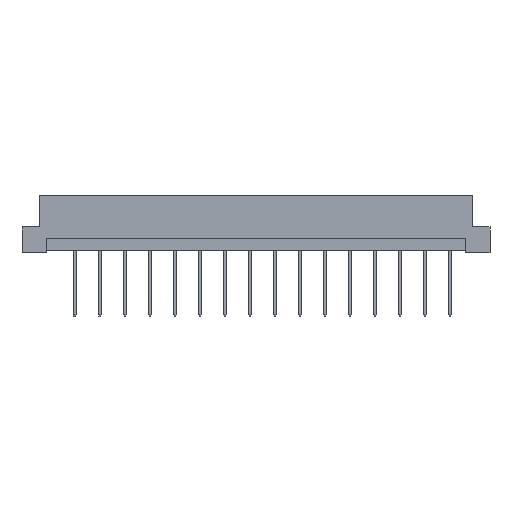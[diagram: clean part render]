
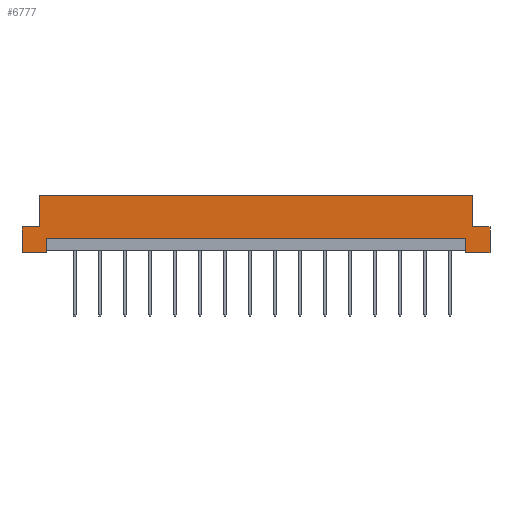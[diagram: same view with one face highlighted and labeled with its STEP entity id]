
A CAD part, front view. The second image highlights one B-rep face of the part: STEP entity #6777.
In plain terms, the highlighted planar face has unit normal (0, -1, 0).
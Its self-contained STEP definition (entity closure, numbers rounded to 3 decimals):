
#1 = VERTEX_POINT ( 'NONE', #7592 ) ;
#35 = EDGE_CURVE ( 'NONE', #4736, #4532, #8822, .T. ) ;
#127 = VERTEX_POINT ( 'NONE', #9904 ) ;
#182 = ORIENTED_EDGE ( 'NONE', *, *, #8289, .F. ) ;
#569 = LINE ( 'NONE', #14402, #5395 ) ;
#640 = VECTOR ( 'NONE', #4607, 1000. ) ;
#718 = VERTEX_POINT ( 'NONE', #14278 ) ;
#789 = DIRECTION ( 'NONE',  ( 0., 0., 1. ) ) ;
#864 = CARTESIAN_POINT ( 'NONE',  ( 44., 0., 5.2 ) ) ;
#945 = EDGE_CURVE ( 'NONE', #718, #7677, #9949, .T. ) ;
#1188 = CARTESIAN_POINT ( 'NONE',  ( -44., 0., 5.2 ) ) ;
#1294 = CARTESIAN_POINT ( 'NONE',  ( -47.5, 0., 0. ) ) ;
#1358 = CARTESIAN_POINT ( 'NONE',  ( 44., 0., 11.6 ) ) ;
#1522 = LINE ( 'NONE', #8984, #9088 ) ;
#1700 = VERTEX_POINT ( 'NONE', #8408 ) ;
#1978 = CARTESIAN_POINT ( 'NONE',  ( -42.6, 0., 2.9 ) ) ;
#1984 = VERTEX_POINT ( 'NONE', #1978 ) ;
#1985 = CARTESIAN_POINT ( 'NONE',  ( -42.6, 0., 0. ) ) ;
#1991 = ORIENTED_EDGE ( 'NONE', *, *, #945, .T. ) ;
#2161 = ORIENTED_EDGE ( 'NONE', *, *, #4704, .F. ) ;
#2225 = DIRECTION ( 'NONE',  ( 1., 0., 0. ) ) ;
#2339 = LINE ( 'NONE', #2666, #5814 ) ;
#2380 = EDGE_LOOP ( 'NONE', ( #9083, #1991, #13119, #13314, #182, #15632, #12056, #8169, #2161, #11505, #4654, #10439 ) ) ;
#2666 = CARTESIAN_POINT ( 'NONE',  ( -47.5, 0., 0. ) ) ;
#2868 = CARTESIAN_POINT ( 'NONE',  ( -44., 0., 5.2 ) ) ;
#3028 = PLANE ( 'NONE',  #11370 ) ;
#3866 = CARTESIAN_POINT ( 'NONE',  ( 47.5, 0., 0. ) ) ;
#4532 = VERTEX_POINT ( 'NONE', #11679 ) ;
#4539 = CARTESIAN_POINT ( 'NONE',  ( 42.6, 0., 0. ) ) ;
#4597 = DIRECTION ( 'NONE',  ( 1., 0., 0. ) ) ;
#4607 = DIRECTION ( 'NONE',  ( -1., 0., 0. ) ) ;
#4654 = ORIENTED_EDGE ( 'NONE', *, *, #35, .F. ) ;
#4704 = EDGE_CURVE ( 'NONE', #1700, #7177, #9771, .T. ) ;
#4736 = VERTEX_POINT ( 'NONE', #1985 ) ;
#5165 = DIRECTION ( 'NONE',  ( 0., 0., -1. ) ) ;
#5188 = EDGE_CURVE ( 'NONE', #718, #1984, #10901, .T. ) ;
#5386 = VECTOR ( 'NONE', #4597, 1000. ) ;
#5395 = VECTOR ( 'NONE', #10674, 1000. ) ;
#5814 = VECTOR ( 'NONE', #10034, 1000. ) ;
#5982 = CARTESIAN_POINT ( 'NONE',  ( 44., 0., 5.2 ) ) ;
#6008 = LINE ( 'NONE', #12214, #5386 ) ;
#6777 = ADVANCED_FACE ( 'NONE', ( #15205 ), #3028, .F. ) ;
#7177 = VERTEX_POINT ( 'NONE', #1188 ) ;
#7311 = CARTESIAN_POINT ( 'NONE',  ( 42.6, 0., 0.5 ) ) ;
#7526 = EDGE_CURVE ( 'NONE', #12437, #7677, #2339, .T. ) ;
#7537 = VECTOR ( 'NONE', #15791, 1000. ) ;
#7592 = CARTESIAN_POINT ( 'NONE',  ( -44., 0., 11.6 ) ) ;
#7677 = VERTEX_POINT ( 'NONE', #4539 ) ;
#7751 = DIRECTION ( 'NONE',  ( -1., 0., 0. ) ) ;
#7992 = CARTESIAN_POINT ( 'NONE',  ( -47.5, 0., 11.6 ) ) ;
#8162 = EDGE_CURVE ( 'NONE', #4532, #1700, #14466, .T. ) ;
#8169 = ORIENTED_EDGE ( 'NONE', *, *, #15074, .F. ) ;
#8289 = EDGE_CURVE ( 'NONE', #15719, #127, #6008, .T. ) ;
#8305 = EDGE_CURVE ( 'NONE', #15719, #9789, #13549, .T. ) ;
#8408 = CARTESIAN_POINT ( 'NONE',  ( -47.5, 0., 5.2 ) ) ;
#8822 = LINE ( 'NONE', #1294, #11582 ) ;
#8984 = CARTESIAN_POINT ( 'NONE',  ( -42.6, 0., 0.5 ) ) ;
#9083 = ORIENTED_EDGE ( 'NONE', *, *, #5188, .F. ) ;
#9088 = VECTOR ( 'NONE', #5165, 1000. ) ;
#9163 = DIRECTION ( 'NONE',  ( 0., 0., 1. ) ) ;
#9628 = CARTESIAN_POINT ( 'NONE',  ( 47.5, 0., 0. ) ) ;
#9720 = LINE ( 'NONE', #9628, #15157 ) ;
#9771 = LINE ( 'NONE', #14647, #16210 ) ;
#9789 = VERTEX_POINT ( 'NONE', #1358 ) ;
#9904 = CARTESIAN_POINT ( 'NONE',  ( 47.5, 0., 5.2 ) ) ;
#9949 = LINE ( 'NONE', #7311, #12386 ) ;
#10034 = DIRECTION ( 'NONE',  ( -1., 0., 0. ) ) ;
#10439 = ORIENTED_EDGE ( 'NONE', *, *, #11643, .F. ) ;
#10487 = LINE ( 'NONE', #2868, #13439 ) ;
#10674 = DIRECTION ( 'NONE',  ( 1., 0., 0. ) ) ;
#10885 = EDGE_CURVE ( 'NONE', #1, #9789, #569, .T. ) ;
#10901 = LINE ( 'NONE', #15948, #640 ) ;
#11370 = AXIS2_PLACEMENT_3D ( 'NONE', #7992, #13055, #9163 ) ;
#11505 = ORIENTED_EDGE ( 'NONE', *, *, #8162, .F. ) ;
#11582 = VECTOR ( 'NONE', #7751, 1000. ) ;
#11643 = EDGE_CURVE ( 'NONE', #1984, #4736, #1522, .T. ) ;
#11679 = CARTESIAN_POINT ( 'NONE',  ( -47.5, 0., 0. ) ) ;
#11767 = EDGE_CURVE ( 'NONE', #127, #12437, #9720, .T. ) ;
#12052 = CARTESIAN_POINT ( 'NONE',  ( -47.5, 0., 0. ) ) ;
#12056 = ORIENTED_EDGE ( 'NONE', *, *, #10885, .F. ) ;
#12214 = CARTESIAN_POINT ( 'NONE',  ( 47.5, 0., 5.2 ) ) ;
#12386 = VECTOR ( 'NONE', #15079, 1000. ) ;
#12437 = VERTEX_POINT ( 'NONE', #3866 ) ;
#13055 = DIRECTION ( 'NONE',  ( 0., 1., 0. ) ) ;
#13119 = ORIENTED_EDGE ( 'NONE', *, *, #7526, .F. ) ;
#13314 = ORIENTED_EDGE ( 'NONE', *, *, #11767, .F. ) ;
#13439 = VECTOR ( 'NONE', #15535, 1000. ) ;
#13549 = LINE ( 'NONE', #864, #14125 ) ;
#14125 = VECTOR ( 'NONE', #789, 1000. ) ;
#14278 = CARTESIAN_POINT ( 'NONE',  ( 42.6, 0., 2.9 ) ) ;
#14402 = CARTESIAN_POINT ( 'NONE',  ( -47.5, 0., 11.6 ) ) ;
#14466 = LINE ( 'NONE', #12052, #7537 ) ;
#14647 = CARTESIAN_POINT ( 'NONE',  ( -47.5, 0., 5.2 ) ) ;
#15006 = DIRECTION ( 'NONE',  ( 0., 0., -1. ) ) ;
#15074 = EDGE_CURVE ( 'NONE', #7177, #1, #10487, .T. ) ;
#15079 = DIRECTION ( 'NONE',  ( 0., 0., -1. ) ) ;
#15157 = VECTOR ( 'NONE', #15006, 1000. ) ;
#15205 = FACE_OUTER_BOUND ( 'NONE', #2380, .T. ) ;
#15535 = DIRECTION ( 'NONE',  ( 0., 0., 1. ) ) ;
#15632 = ORIENTED_EDGE ( 'NONE', *, *, #8305, .T. ) ;
#15719 = VERTEX_POINT ( 'NONE', #5982 ) ;
#15791 = DIRECTION ( 'NONE',  ( 0., 0., 1. ) ) ;
#15948 = CARTESIAN_POINT ( 'NONE',  ( 42.6, 0., 2.9 ) ) ;
#16210 = VECTOR ( 'NONE', #2225, 1000. ) ;
